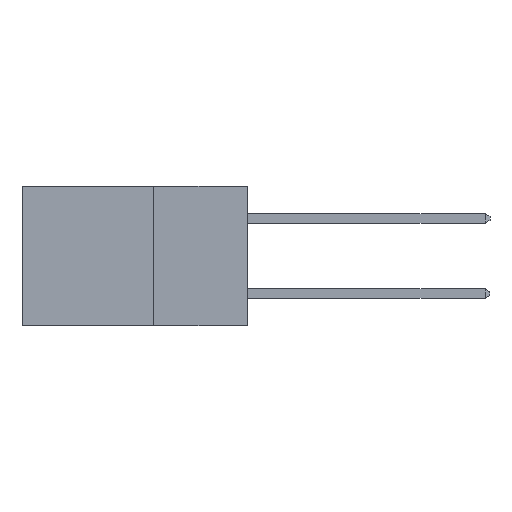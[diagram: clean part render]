
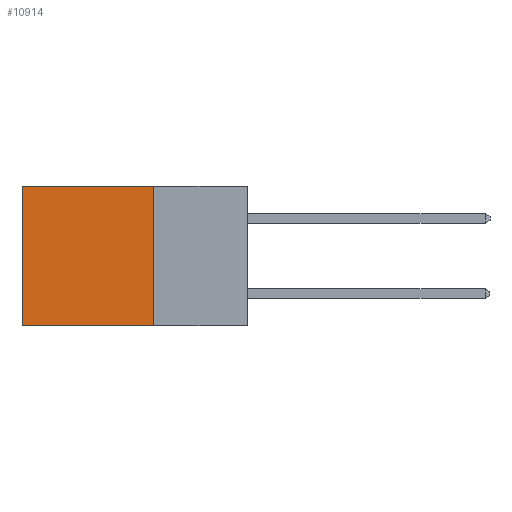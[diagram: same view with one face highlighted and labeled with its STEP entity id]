
A CAD part, left-side view. The second image highlights one B-rep face of the part: STEP entity #10914.
In plain terms, the highlighted planar face has unit normal (-1, 0, 0).
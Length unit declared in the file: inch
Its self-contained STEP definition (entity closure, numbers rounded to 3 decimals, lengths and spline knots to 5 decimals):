
#1117 = VECTOR ( 'NONE', #2572, 39.37008 ) ;
#1152 = ORIENTED_EDGE ( 'NONE', *, *, #3216, .F. ) ;
#1660 = EDGE_LOOP ( 'NONE', ( #4789, #10829, #1152, #2029 ) ) ;
#1873 = EDGE_CURVE ( 'NONE', #10070, #11786, #10031, .T. ) ;
#1918 = CARTESIAN_POINT ( 'NONE',  ( 0.298, 0.25, 0. ) ) ;
#1981 = VERTEX_POINT ( 'NONE', #4888 ) ;
#2029 = ORIENTED_EDGE ( 'NONE', *, *, #12775, .T. ) ;
#2377 = AXIS2_PLACEMENT_3D ( 'NONE', #2692, #10205, #3854 ) ;
#2384 = CARTESIAN_POINT ( 'NONE',  ( 0.298, 0.25, -0.37 ) ) ;
#2572 = DIRECTION ( 'NONE',  ( 0., 1., 0. ) ) ;
#2585 = CARTESIAN_POINT ( 'NONE',  ( 0.298, 0.6, 0. ) ) ;
#2692 = CARTESIAN_POINT ( 'NONE',  ( 0.298, 0.25, 0. ) ) ;
#2697 = FACE_OUTER_BOUND ( 'NONE', #1660, .T. ) ;
#3216 = EDGE_CURVE ( 'NONE', #1981, #5689, #9092, .T. ) ;
#3854 = DIRECTION ( 'NONE',  ( 0., 0., -1. ) ) ;
#4243 = DIRECTION ( 'NONE',  ( 0., 0., -1. ) ) ;
#4342 = EDGE_CURVE ( 'NONE', #5689, #11786, #7109, .T. ) ;
#4390 = VECTOR ( 'NONE', #4243, 39.37008 ) ;
#4789 = ORIENTED_EDGE ( 'NONE', *, *, #1873, .T. ) ;
#4888 = CARTESIAN_POINT ( 'NONE',  ( 0.298, 0.25, 0. ) ) ;
#5689 = VERTEX_POINT ( 'NONE', #5985 ) ;
#5985 = CARTESIAN_POINT ( 'NONE',  ( 0.298, 0.25, -0.37 ) ) ;
#6298 = VECTOR ( 'NONE', #12319, 39.37008 ) ;
#6462 = VECTOR ( 'NONE', #10631, 39.37008 ) ;
#7109 = LINE ( 'NONE', #2384, #1117 ) ;
#8442 = CARTESIAN_POINT ( 'NONE',  ( 0.298, 0.6, -0.37 ) ) ;
#8614 = CARTESIAN_POINT ( 'NONE',  ( 0.298, 0.25, 0. ) ) ;
#9092 = LINE ( 'NONE', #1918, #6298 ) ;
#9234 = LINE ( 'NONE', #8614, #6462 ) ;
#10031 = LINE ( 'NONE', #2585, #4390 ) ;
#10070 = VERTEX_POINT ( 'NONE', #12850 ) ;
#10205 = DIRECTION ( 'NONE',  ( 1., 0., 0. ) ) ;
#10631 = DIRECTION ( 'NONE',  ( 0., 1., 0. ) ) ;
#10829 = ORIENTED_EDGE ( 'NONE', *, *, #4342, .F. ) ;
#10914 = ADVANCED_FACE ( 'NONE', ( #2697 ), #13190, .F. ) ;
#11786 = VERTEX_POINT ( 'NONE', #8442 ) ;
#12319 = DIRECTION ( 'NONE',  ( 0., 0., -1. ) ) ;
#12775 = EDGE_CURVE ( 'NONE', #1981, #10070, #9234, .T. ) ;
#12850 = CARTESIAN_POINT ( 'NONE',  ( 0.298, 0.6, 0. ) ) ;
#13190 = PLANE ( 'NONE',  #2377 ) ;
